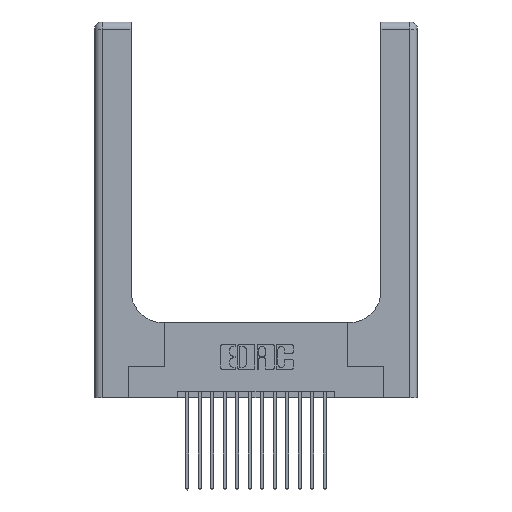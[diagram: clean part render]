
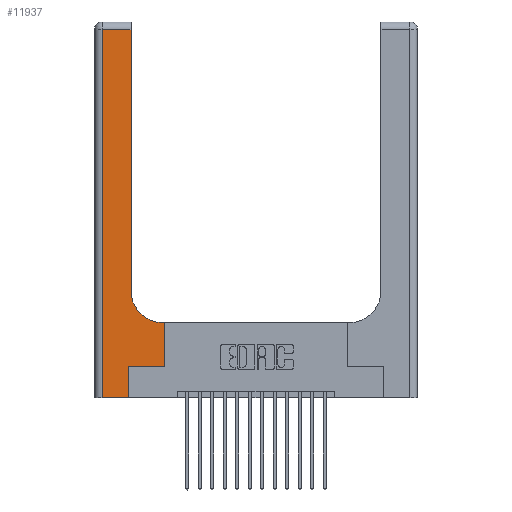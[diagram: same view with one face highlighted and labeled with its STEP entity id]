
A CAD part, top view. The second image highlights one B-rep face of the part: STEP entity #11937.
In plain terms, the highlighted planar face has unit normal (0, 0, 1).
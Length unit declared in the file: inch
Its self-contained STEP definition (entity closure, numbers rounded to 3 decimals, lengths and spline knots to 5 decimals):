
#231 = EDGE_CURVE ( 'NONE', #6746, #11977, #9078, .T. ) ;
#289 = DIRECTION ( 'NONE',  ( -1., 0., 0. ) ) ;
#719 = AXIS2_PLACEMENT_3D ( 'NONE', #2439, #18380, #16922 ) ;
#966 = CARTESIAN_POINT ( 'NONE',  ( 0., 0., 0.37 ) ) ;
#1050 = CARTESIAN_POINT ( 'NONE',  ( 0.5585, 0.25, 0.37 ) ) ;
#1419 = CARTESIAN_POINT ( 'NONE',  ( 0.269, 0.25, 0.37 ) ) ;
#1466 = VERTEX_POINT ( 'NONE', #18157 ) ;
#1989 = EDGE_CURVE ( 'NONE', #14194, #6746, #14437, .T. ) ;
#2043 = EDGE_CURVE ( 'NONE', #18054, #2580, #14860, .T. ) ;
#2058 = LINE ( 'NONE', #1050, #16729 ) ;
#2439 = CARTESIAN_POINT ( 'NONE',  ( 0., 3., 0.37 ) ) ;
#2580 = VERTEX_POINT ( 'NONE', #12041 ) ;
#4192 = CARTESIAN_POINT ( 'NONE',  ( 0.06, 3., 0.37 ) ) ;
#4640 = ORIENTED_EDGE ( 'NONE', *, *, #14836, .T. ) ;
#4783 = CARTESIAN_POINT ( 'NONE',  ( 0.2915, 0.85, 0.37 ) ) ;
#4880 = DIRECTION ( 'NONE',  ( -1., 0., 0. ) ) ;
#4943 = CARTESIAN_POINT ( 'NONE',  ( 0.2915, 3., 0.37 ) ) ;
#5024 = DIRECTION ( 'NONE',  ( 1., 0., 0. ) ) ;
#5179 = VECTOR ( 'NONE', #4880, 39.37008 ) ;
#5475 = AXIS2_PLACEMENT_3D ( 'NONE', #11018, #6407, #5024 ) ;
#6311 = VECTOR ( 'NONE', #13593, 39.37008 ) ;
#6407 = DIRECTION ( 'NONE',  ( 0., 0., -1. ) ) ;
#6538 = ORIENTED_EDGE ( 'NONE', *, *, #1989, .T. ) ;
#6746 = VERTEX_POINT ( 'NONE', #8081 ) ;
#7216 = FACE_OUTER_BOUND ( 'NONE', #8539, .T. ) ;
#7982 = LINE ( 'NONE', #4192, #16998 ) ;
#8081 = CARTESIAN_POINT ( 'NONE',  ( 0.2915, 2.94, 0.37 ) ) ;
#8105 = DIRECTION ( 'NONE',  ( 1., 0., 0. ) ) ;
#8361 = DIRECTION ( 'NONE',  ( 0., -1., 0. ) ) ;
#8414 = LINE ( 'NONE', #9748, #17914 ) ;
#8539 = EDGE_LOOP ( 'NONE', ( #6538, #8617, #9110, #10263, #16410, #13335, #11793, #12317, #4640 ) ) ;
#8617 = ORIENTED_EDGE ( 'NONE', *, *, #231, .T. ) ;
#9078 = LINE ( 'NONE', #10264, #11118 ) ;
#9110 = ORIENTED_EDGE ( 'NONE', *, *, #9883, .T. ) ;
#9748 = CARTESIAN_POINT ( 'NONE',  ( 0.269, 0., 0.37 ) ) ;
#9795 = PLANE ( 'NONE',  #719 ) ;
#9802 = VERTEX_POINT ( 'NONE', #16764 ) ;
#9883 = EDGE_CURVE ( 'NONE', #11977, #9802, #7982, .T. ) ;
#9939 = EDGE_CURVE ( 'NONE', #14095, #1466, #8414, .T. ) ;
#10076 = LINE ( 'NONE', #966, #13480 ) ;
#10263 = ORIENTED_EDGE ( 'NONE', *, *, #13908, .T. ) ;
#10264 = CARTESIAN_POINT ( 'NONE',  ( 0., 2.94, 0.37 ) ) ;
#10756 = CARTESIAN_POINT ( 'NONE',  ( 0.2915, 0.6, 0.37 ) ) ;
#11018 = CARTESIAN_POINT ( 'NONE',  ( 0.5415, 0.85, 0.37 ) ) ;
#11066 = DIRECTION ( 'NONE',  ( 0., 1., 0. ) ) ;
#11118 = VECTOR ( 'NONE', #289, 39.37008 ) ;
#11793 = ORIENTED_EDGE ( 'NONE', *, *, #18062, .T. ) ;
#11937 = ADVANCED_FACE ( 'NONE', ( #7216 ), #9795, .F. ) ;
#11977 = VERTEX_POINT ( 'NONE', #18554 ) ;
#12041 = CARTESIAN_POINT ( 'NONE',  ( 0.5415, 0.6, 0.37 ) ) ;
#12317 = ORIENTED_EDGE ( 'NONE', *, *, #2043, .T. ) ;
#13053 = CARTESIAN_POINT ( 'NONE',  ( 0.269, 0., 0.37 ) ) ;
#13335 = ORIENTED_EDGE ( 'NONE', *, *, #15157, .T. ) ;
#13480 = VECTOR ( 'NONE', #8105, 39.37008 ) ;
#13593 = DIRECTION ( 'NONE',  ( 0., 1., 0. ) ) ;
#13908 = EDGE_CURVE ( 'NONE', #9802, #14095, #10076, .T. ) ;
#14095 = VERTEX_POINT ( 'NONE', #13053 ) ;
#14194 = VERTEX_POINT ( 'NONE', #4783 ) ;
#14437 = LINE ( 'NONE', #4943, #6311 ) ;
#14836 = EDGE_CURVE ( 'NONE', #2580, #14194, #17046, .T. ) ;
#14860 = LINE ( 'NONE', #10756, #5179 ) ;
#15157 = EDGE_CURVE ( 'NONE', #1466, #16894, #18166, .T. ) ;
#15222 = VECTOR ( 'NONE', #17113, 39.37008 ) ;
#16410 = ORIENTED_EDGE ( 'NONE', *, *, #9939, .T. ) ;
#16729 = VECTOR ( 'NONE', #16872, 39.37008 ) ;
#16764 = CARTESIAN_POINT ( 'NONE',  ( 0.06, 0., 0.37 ) ) ;
#16808 = CARTESIAN_POINT ( 'NONE',  ( 0.5585, 0.6, 0.37 ) ) ;
#16872 = DIRECTION ( 'NONE',  ( 0., 1., 0. ) ) ;
#16894 = VERTEX_POINT ( 'NONE', #17086 ) ;
#16922 = DIRECTION ( 'NONE',  ( -1., 0., 0. ) ) ;
#16998 = VECTOR ( 'NONE', #8361, 39.37008 ) ;
#17046 = CIRCLE ( 'NONE', #5475, 0.25 ) ;
#17086 = CARTESIAN_POINT ( 'NONE',  ( 0.5585, 0.25, 0.37 ) ) ;
#17113 = DIRECTION ( 'NONE',  ( 1., 0., 0. ) ) ;
#17914 = VECTOR ( 'NONE', #11066, 39.37008 ) ;
#18054 = VERTEX_POINT ( 'NONE', #16808 ) ;
#18062 = EDGE_CURVE ( 'NONE', #16894, #18054, #2058, .T. ) ;
#18157 = CARTESIAN_POINT ( 'NONE',  ( 0.269, 0.25, 0.37 ) ) ;
#18166 = LINE ( 'NONE', #1419, #15222 ) ;
#18380 = DIRECTION ( 'NONE',  ( 0., 0., -1. ) ) ;
#18554 = CARTESIAN_POINT ( 'NONE',  ( 0.06, 2.94, 0.37 ) ) ;
